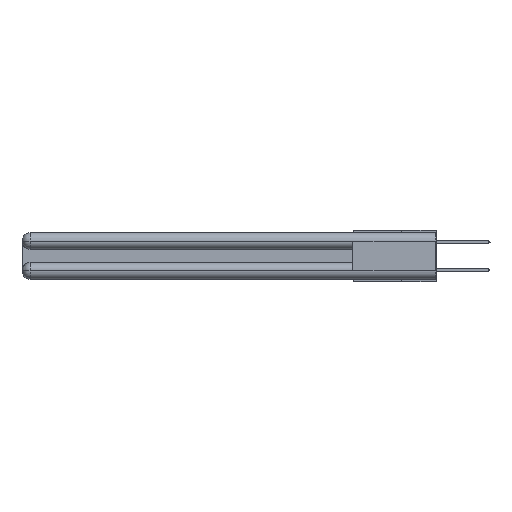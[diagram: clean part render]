
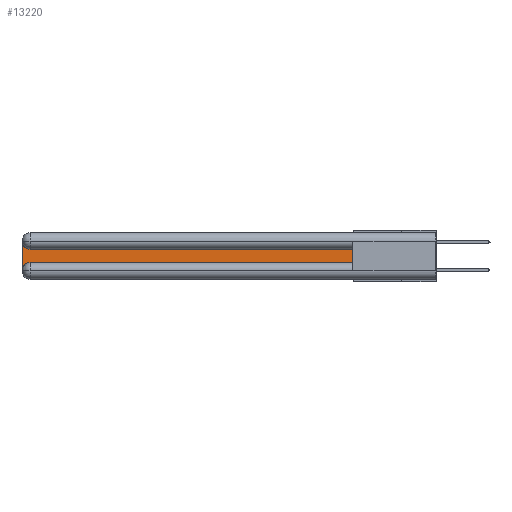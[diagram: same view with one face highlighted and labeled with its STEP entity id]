
A CAD part, left-side view. The second image highlights one B-rep face of the part: STEP entity #13220.
In plain terms, the highlighted planar face has unit normal (-1, 0, 0).
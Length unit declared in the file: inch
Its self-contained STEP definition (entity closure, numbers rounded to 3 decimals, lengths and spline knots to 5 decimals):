
#227 = DIRECTION ( 'NONE',  ( 0., -1., 0. ) ) ;
#703 = CARTESIAN_POINT ( 'NONE',  ( 0.075, 0.6, -0.1225 ) ) ;
#1291 = CIRCLE ( 'NONE', #16278, 0.06 ) ;
#2311 = VECTOR ( 'NONE', #10769, 39.37008 ) ;
#2336 = AXIS2_PLACEMENT_3D ( 'NONE', #16385, #14134, #29004 ) ;
#2505 = EDGE_CURVE ( 'NONE', #9897, #24729, #1291, .T. ) ;
#3780 = VECTOR ( 'NONE', #227, 39.37008 ) ;
#5425 = EDGE_CURVE ( 'NONE', #24729, #26873, #28904, .T. ) ;
#7118 = ORIENTED_EDGE ( 'NONE', *, *, #23061, .T. ) ;
#7898 = EDGE_LOOP ( 'NONE', ( #31904, #13809, #7118, #26732, #18532, #16811 ) ) ;
#8773 = CARTESIAN_POINT ( 'NONE',  ( 0.075, 3., -0.1225 ) ) ;
#8779 = CARTESIAN_POINT ( 'NONE',  ( 0.075, 3., -0.2175 ) ) ;
#8925 = CARTESIAN_POINT ( 'NONE',  ( 0.075, 0.6, -0.2175 ) ) ;
#8988 = DIRECTION ( 'NONE',  ( 0., 0., -1. ) ) ;
#9408 = CIRCLE ( 'NONE', #2336, 0.06 ) ;
#9534 = VERTEX_POINT ( 'NONE', #11875 ) ;
#9607 = EDGE_CURVE ( 'NONE', #30313, #9534, #9408, .T. ) ;
#9897 = VERTEX_POINT ( 'NONE', #24773 ) ;
#10022 = DIRECTION ( 'NONE',  ( 0., 0., 1. ) ) ;
#10769 = DIRECTION ( 'NONE',  ( 0., 1., 0. ) ) ;
#11409 = FACE_OUTER_BOUND ( 'NONE', #7898, .T. ) ;
#11602 = CARTESIAN_POINT ( 'NONE',  ( 0.075, 2.94, -0.2775 ) ) ;
#11875 = CARTESIAN_POINT ( 'NONE',  ( 0.075, 3., -0.0625 ) ) ;
#13220 = ADVANCED_FACE ( 'NONE', ( #11409 ), #18783, .F. ) ;
#13809 = ORIENTED_EDGE ( 'NONE', *, *, #9607, .T. ) ;
#14134 = DIRECTION ( 'NONE',  ( 1., 0., 0. ) ) ;
#14967 = LINE ( 'NONE', #8779, #27667 ) ;
#15207 = CARTESIAN_POINT ( 'NONE',  ( 0.075, 0.6, -0.1225 ) ) ;
#16018 = CARTESIAN_POINT ( 'NONE',  ( 0.075, 2.94, -0.1225 ) ) ;
#16278 = AXIS2_PLACEMENT_3D ( 'NONE', #11602, #26977, #27079 ) ;
#16385 = CARTESIAN_POINT ( 'NONE',  ( 0.075, 2.94, -0.0625 ) ) ;
#16404 = CARTESIAN_POINT ( 'NONE',  ( 0.075, 2.94, -0.2175 ) ) ;
#16585 = VECTOR ( 'NONE', #10022, 39.37008 ) ;
#16811 = ORIENTED_EDGE ( 'NONE', *, *, #17145, .T. ) ;
#17145 = EDGE_CURVE ( 'NONE', #26873, #17212, #30841, .T. ) ;
#17212 = VERTEX_POINT ( 'NONE', #15207 ) ;
#18251 = DIRECTION ( 'NONE',  ( 0., 0., -1. ) ) ;
#18532 = ORIENTED_EDGE ( 'NONE', *, *, #5425, .T. ) ;
#18783 = PLANE ( 'NONE',  #26965 ) ;
#21281 = DIRECTION ( 'NONE',  ( 1., 0., 0. ) ) ;
#21680 = CARTESIAN_POINT ( 'NONE',  ( 0.075, 0.6, -0.2175 ) ) ;
#23061 = EDGE_CURVE ( 'NONE', #9534, #9897, #14967, .T. ) ;
#24437 = CARTESIAN_POINT ( 'NONE',  ( 0.075, 0.6, -0.2175 ) ) ;
#24729 = VERTEX_POINT ( 'NONE', #16404 ) ;
#24773 = CARTESIAN_POINT ( 'NONE',  ( 0.075, 3., -0.2775 ) ) ;
#25077 = EDGE_CURVE ( 'NONE', #17212, #30313, #28554, .T. ) ;
#26732 = ORIENTED_EDGE ( 'NONE', *, *, #2505, .T. ) ;
#26873 = VERTEX_POINT ( 'NONE', #8925 ) ;
#26965 = AXIS2_PLACEMENT_3D ( 'NONE', #8773, #21281, #8988 ) ;
#26977 = DIRECTION ( 'NONE',  ( 1., 0., 0. ) ) ;
#27079 = DIRECTION ( 'NONE',  ( 0., 0., -1. ) ) ;
#27667 = VECTOR ( 'NONE', #18251, 39.37008 ) ;
#28554 = LINE ( 'NONE', #703, #2311 ) ;
#28904 = LINE ( 'NONE', #24437, #3780 ) ;
#29004 = DIRECTION ( 'NONE',  ( 0., 0., -1. ) ) ;
#30313 = VERTEX_POINT ( 'NONE', #16018 ) ;
#30841 = LINE ( 'NONE', #21680, #16585 ) ;
#31904 = ORIENTED_EDGE ( 'NONE', *, *, #25077, .T. ) ;
